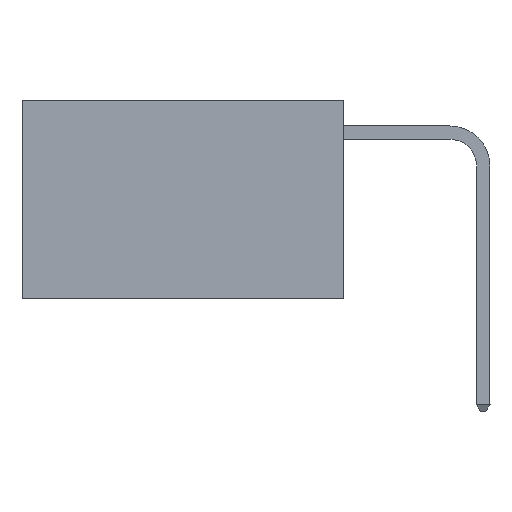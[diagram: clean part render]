
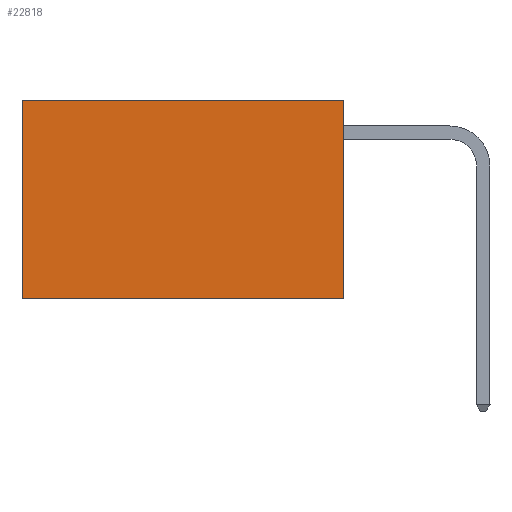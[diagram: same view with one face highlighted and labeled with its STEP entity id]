
A CAD part, left-side view. The second image highlights one B-rep face of the part: STEP entity #22818.
In plain terms, the highlighted planar face has unit normal (-1, 0, 0).
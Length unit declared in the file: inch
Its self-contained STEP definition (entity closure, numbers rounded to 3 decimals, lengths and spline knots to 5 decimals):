
#702 = EDGE_LOOP ( 'NONE', ( #6849, #12679, #11667, #9745 ) ) ;
#809 = DIRECTION ( 'NONE',  ( 0., 1., 0. ) ) ;
#1793 = CARTESIAN_POINT ( 'NONE',  ( 0.2625, 0.6, 0. ) ) ;
#3080 = FACE_OUTER_BOUND ( 'NONE', #702, .T. ) ;
#3233 = CARTESIAN_POINT ( 'NONE',  ( 0.2625, 0., -0.37 ) ) ;
#3471 = CARTESIAN_POINT ( 'NONE',  ( 0.2625, 0.6, 0. ) ) ;
#4164 = VERTEX_POINT ( 'NONE', #3233 ) ;
#4561 = CARTESIAN_POINT ( 'NONE',  ( 0.2625, 0., 0. ) ) ;
#5491 = LINE ( 'NONE', #9118, #28477 ) ;
#6202 = DIRECTION ( 'NONE',  ( 0., 0., -1. ) ) ;
#6248 = EDGE_CURVE ( 'NONE', #17266, #20082, #8012, .T. ) ;
#6849 = ORIENTED_EDGE ( 'NONE', *, *, #6248, .T. ) ;
#7393 = DIRECTION ( 'NONE',  ( 0., 0., -1. ) ) ;
#8012 = LINE ( 'NONE', #1793, #25085 ) ;
#8134 = PLANE ( 'NONE',  #23758 ) ;
#9118 = CARTESIAN_POINT ( 'NONE',  ( 0.2625, 0., -0.37 ) ) ;
#9633 = VERTEX_POINT ( 'NONE', #4561 ) ;
#9745 = ORIENTED_EDGE ( 'NONE', *, *, #22585, .T. ) ;
#10062 = CARTESIAN_POINT ( 'NONE',  ( 0.2625, 0.6, -0.37 ) ) ;
#11667 = ORIENTED_EDGE ( 'NONE', *, *, #21868, .F. ) ;
#11789 = LINE ( 'NONE', #22974, #27492 ) ;
#11849 = CARTESIAN_POINT ( 'NONE',  ( 0.2625, 0., 0. ) ) ;
#12638 = DIRECTION ( 'NONE',  ( 0., 0., -1. ) ) ;
#12679 = ORIENTED_EDGE ( 'NONE', *, *, #22476, .F. ) ;
#14569 = LINE ( 'NONE', #11849, #19757 ) ;
#17266 = VERTEX_POINT ( 'NONE', #3471 ) ;
#19757 = VECTOR ( 'NONE', #809, 39.37008 ) ;
#20082 = VERTEX_POINT ( 'NONE', #10062 ) ;
#21868 = EDGE_CURVE ( 'NONE', #9633, #4164, #11789, .T. ) ;
#22476 = EDGE_CURVE ( 'NONE', #4164, #20082, #5491, .T. ) ;
#22585 = EDGE_CURVE ( 'NONE', #9633, #17266, #14569, .T. ) ;
#22818 = ADVANCED_FACE ( 'NONE', ( #3080 ), #8134, .F. ) ;
#22974 = CARTESIAN_POINT ( 'NONE',  ( 0.2625, 0., 0. ) ) ;
#23711 = CARTESIAN_POINT ( 'NONE',  ( 0.2625, 0., 0. ) ) ;
#23758 = AXIS2_PLACEMENT_3D ( 'NONE', #23711, #25953, #12638 ) ;
#24808 = DIRECTION ( 'NONE',  ( 0., 1., 0. ) ) ;
#25085 = VECTOR ( 'NONE', #6202, 39.37008 ) ;
#25953 = DIRECTION ( 'NONE',  ( 1., 0., 0. ) ) ;
#27492 = VECTOR ( 'NONE', #7393, 39.37008 ) ;
#28477 = VECTOR ( 'NONE', #24808, 39.37008 ) ;
